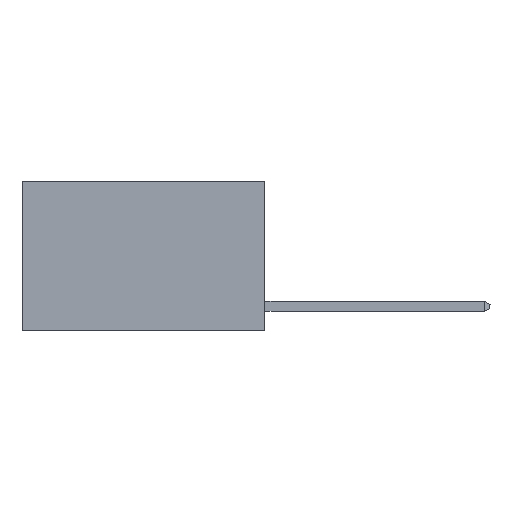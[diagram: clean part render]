
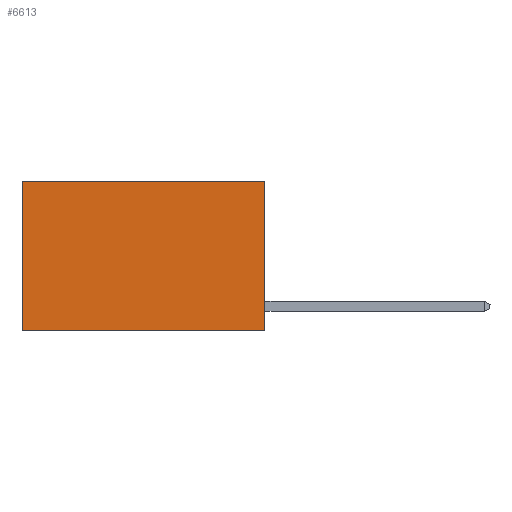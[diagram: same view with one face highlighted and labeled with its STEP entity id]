
A CAD part, left-side view. The second image highlights one B-rep face of the part: STEP entity #6613.
In plain terms, the highlighted planar face has unit normal (-1, 0, 0).
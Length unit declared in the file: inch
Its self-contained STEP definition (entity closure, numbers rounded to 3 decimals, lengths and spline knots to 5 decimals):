
#592 = AXIS2_PLACEMENT_3D ( 'NONE', #843, #6155, #18155 ) ;
#843 = CARTESIAN_POINT ( 'NONE',  ( 0.2625, 0., 0. ) ) ;
#1199 = CARTESIAN_POINT ( 'NONE',  ( 0.2625, 0.6, -0.37 ) ) ;
#1375 = FACE_OUTER_BOUND ( 'NONE', #5311, .T. ) ;
#1951 = LINE ( 'NONE', #8559, #10145 ) ;
#2950 = ORIENTED_EDGE ( 'NONE', *, *, #21458, .T. ) ;
#3694 = CARTESIAN_POINT ( 'NONE',  ( 0.2625, 0., 0. ) ) ;
#3751 = ORIENTED_EDGE ( 'NONE', *, *, #6211, .F. ) ;
#4381 = PLANE ( 'NONE',  #592 ) ;
#4561 = LINE ( 'NONE', #13846, #13772 ) ;
#4630 = VERTEX_POINT ( 'NONE', #14451 ) ;
#5311 = EDGE_LOOP ( 'NONE', ( #2950, #16018, #3751, #6828 ) ) ;
#5388 = VERTEX_POINT ( 'NONE', #1199 ) ;
#6155 = DIRECTION ( 'NONE',  ( 1., 0., 0. ) ) ;
#6211 = EDGE_CURVE ( 'NONE', #17056, #4630, #1951, .T. ) ;
#6308 = CARTESIAN_POINT ( 'NONE',  ( 0.2625, 0.6, 0. ) ) ;
#6613 = ADVANCED_FACE ( 'NONE', ( #1375 ), #4381, .F. ) ;
#6828 = ORIENTED_EDGE ( 'NONE', *, *, #16980, .T. ) ;
#7624 = VECTOR ( 'NONE', #8070, 39.37008 ) ;
#8070 = DIRECTION ( 'NONE',  ( 0., 0., -1. ) ) ;
#8559 = CARTESIAN_POINT ( 'NONE',  ( 0.2625, 0., 0. ) ) ;
#9254 = DIRECTION ( 'NONE',  ( 0., 1., 0. ) ) ;
#10145 = VECTOR ( 'NONE', #10253, 39.37008 ) ;
#10253 = DIRECTION ( 'NONE',  ( 0., 0., -1. ) ) ;
#10889 = CARTESIAN_POINT ( 'NONE',  ( 0.2625, 0., -0.37 ) ) ;
#11305 = VECTOR ( 'NONE', #9254, 39.37008 ) ;
#11848 = LINE ( 'NONE', #10889, #11305 ) ;
#13772 = VECTOR ( 'NONE', #17263, 39.37008 ) ;
#13846 = CARTESIAN_POINT ( 'NONE',  ( 0.2625, 0., 0. ) ) ;
#14451 = CARTESIAN_POINT ( 'NONE',  ( 0.2625, 0., -0.37 ) ) ;
#15291 = CARTESIAN_POINT ( 'NONE',  ( 0.2625, 0.6, 0. ) ) ;
#16018 = ORIENTED_EDGE ( 'NONE', *, *, #17716, .F. ) ;
#16980 = EDGE_CURVE ( 'NONE', #17056, #21731, #4561, .T. ) ;
#17056 = VERTEX_POINT ( 'NONE', #3694 ) ;
#17263 = DIRECTION ( 'NONE',  ( 0., 1., 0. ) ) ;
#17716 = EDGE_CURVE ( 'NONE', #4630, #5388, #11848, .T. ) ;
#18155 = DIRECTION ( 'NONE',  ( 0., 0., -1. ) ) ;
#21302 = LINE ( 'NONE', #6308, #7624 ) ;
#21458 = EDGE_CURVE ( 'NONE', #21731, #5388, #21302, .T. ) ;
#21731 = VERTEX_POINT ( 'NONE', #15291 ) ;
